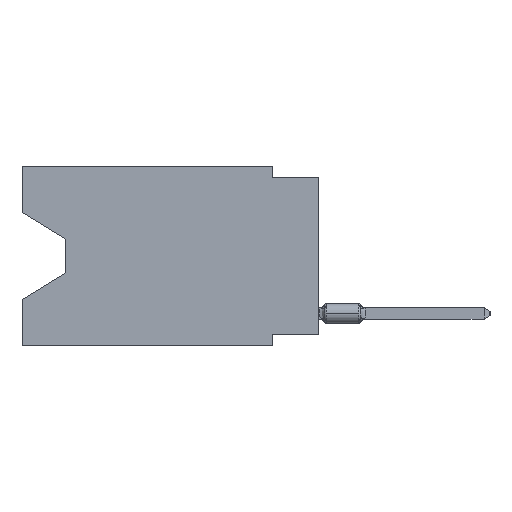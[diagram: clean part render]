
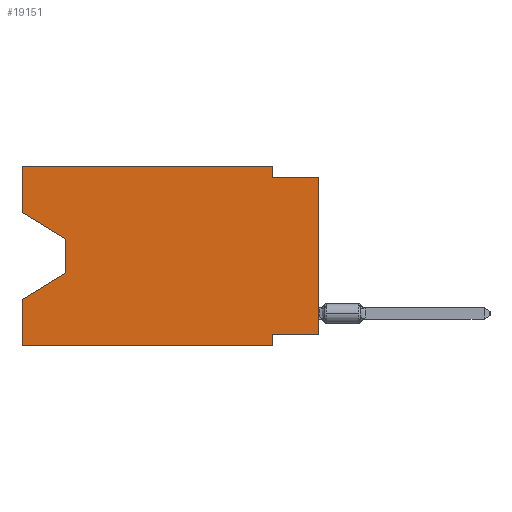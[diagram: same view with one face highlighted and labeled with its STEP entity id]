
A CAD part, left-side view. The second image highlights one B-rep face of the part: STEP entity #19151.
In plain terms, the highlighted planar face has unit normal (-1, 0, 0).
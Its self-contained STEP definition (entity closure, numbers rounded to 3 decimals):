
#124 = CARTESIAN_POINT ( 'NONE',  ( 0., 2.54, -0.635 ) ) ;
#168 = VECTOR ( 'NONE', #8732, 1000. ) ;
#340 = CARTESIAN_POINT ( 'NONE',  ( 0., 2.54, 0. ) ) ;
#761 = CARTESIAN_POINT ( 'NONE',  ( 0., 2.54, -9.271 ) ) ;
#999 = EDGE_CURVE ( 'NONE', #3724, #24567, #1576, .T. ) ;
#1159 = LINE ( 'NONE', #17522, #9940 ) ;
#1576 = LINE ( 'NONE', #15532, #2021 ) ;
#2021 = VECTOR ( 'NONE', #21964, 1000. ) ;
#2259 = VECTOR ( 'NONE', #9205, 1000. ) ;
#2553 = CARTESIAN_POINT ( 'NONE',  ( 0., 16.383, 0. ) ) ;
#3724 = VERTEX_POINT ( 'NONE', #340 ) ;
#3822 = VERTEX_POINT ( 'NONE', #23517 ) ;
#3985 = CARTESIAN_POINT ( 'NONE',  ( 0., 13.97, -4.013 ) ) ;
#4241 = EDGE_CURVE ( 'NONE', #12847, #3724, #4592, .T. ) ;
#4518 = CARTESIAN_POINT ( 'NONE',  ( 0., 16.383, 0. ) ) ;
#4592 = LINE ( 'NONE', #2553, #168 ) ;
#4938 = AXIS2_PLACEMENT_3D ( 'NONE', #4518, #24646, #8543 ) ;
#5073 = VERTEX_POINT ( 'NONE', #761 ) ;
#5089 = EDGE_CURVE ( 'NONE', #18502, #16175, #13225, .T. ) ;
#5400 = EDGE_CURVE ( 'NONE', #19170, #5073, #24892, .T. ) ;
#6096 = DIRECTION ( 'NONE',  ( 0., -0.855, -0.519 ) ) ;
#6120 = DIRECTION ( 'NONE',  ( 0., 0., -1. ) ) ;
#6933 = VECTOR ( 'NONE', #7086, 1000. ) ;
#7086 = DIRECTION ( 'NONE',  ( 0., -1., 0. ) ) ;
#7178 = EDGE_LOOP ( 'NONE', ( #16000, #24976, #16174, #12053, #7689, #14075, #20130, #25928, #21054, #15709, #17109, #22818 ) ) ;
#7386 = CARTESIAN_POINT ( 'NONE',  ( 0., 16.383, 0. ) ) ;
#7527 = VECTOR ( 'NONE', #6096, 1000. ) ;
#7684 = DIRECTION ( 'NONE',  ( 0., -1., 0. ) ) ;
#7689 = ORIENTED_EDGE ( 'NONE', *, *, #8648, .T. ) ;
#8277 = PLANE ( 'NONE',  #4938 ) ;
#8543 = DIRECTION ( 'NONE',  ( 0., 0., -1. ) ) ;
#8648 = EDGE_CURVE ( 'NONE', #18502, #16635, #19505, .T. ) ;
#8732 = DIRECTION ( 'NONE',  ( 0., -1., 0. ) ) ;
#9083 = LINE ( 'NONE', #25455, #6933 ) ;
#9205 = DIRECTION ( 'NONE',  ( 0., 0., 1. ) ) ;
#9466 = CARTESIAN_POINT ( 'NONE',  ( 0., 16.383, 0. ) ) ;
#9786 = CARTESIAN_POINT ( 'NONE',  ( 0., 0., 0. ) ) ;
#9940 = VECTOR ( 'NONE', #11191, 1000. ) ;
#9993 = LINE ( 'NONE', #14555, #7527 ) ;
#11191 = DIRECTION ( 'NONE',  ( 0., 0., 1. ) ) ;
#11523 = DIRECTION ( 'NONE',  ( 0., 0., 1. ) ) ;
#11821 = CARTESIAN_POINT ( 'NONE',  ( 0., 16.383, -9.906 ) ) ;
#12053 = ORIENTED_EDGE ( 'NONE', *, *, #5089, .F. ) ;
#12278 = EDGE_CURVE ( 'NONE', #24567, #22114, #9083, .T. ) ;
#12280 = EDGE_CURVE ( 'NONE', #24946, #16175, #23456, .T. ) ;
#12535 = EDGE_CURVE ( 'NONE', #22841, #12847, #1159, .T. ) ;
#12847 = VERTEX_POINT ( 'NONE', #7386 ) ;
#13225 = LINE ( 'NONE', #9466, #2259 ) ;
#13651 = DIRECTION ( 'NONE',  ( 0., 0.855, -0.519 ) ) ;
#13771 = CARTESIAN_POINT ( 'NONE',  ( 0., 13.97, -5.893 ) ) ;
#14075 = ORIENTED_EDGE ( 'NONE', *, *, #21015, .F. ) ;
#14244 = VECTOR ( 'NONE', #13651, 1000. ) ;
#14555 = CARTESIAN_POINT ( 'NONE',  ( 0., 16.383, -2.546 ) ) ;
#15532 = CARTESIAN_POINT ( 'NONE',  ( 0., 2.54, 0. ) ) ;
#15672 = CARTESIAN_POINT ( 'NONE',  ( 0., 0., -0.635 ) ) ;
#15709 = ORIENTED_EDGE ( 'NONE', *, *, #999, .F. ) ;
#16000 = ORIENTED_EDGE ( 'NONE', *, *, #19570, .T. ) ;
#16169 = CARTESIAN_POINT ( 'NONE',  ( 0., 2.54, -9.906 ) ) ;
#16174 = ORIENTED_EDGE ( 'NONE', *, *, #12280, .T. ) ;
#16175 = VERTEX_POINT ( 'NONE', #18248 ) ;
#16287 = LINE ( 'NONE', #16169, #22493 ) ;
#16613 = FACE_OUTER_BOUND ( 'NONE', #7178, .T. ) ;
#16635 = VERTEX_POINT ( 'NONE', #26372 ) ;
#17109 = ORIENTED_EDGE ( 'NONE', *, *, #4241, .F. ) ;
#17522 = CARTESIAN_POINT ( 'NONE',  ( 0., 16.383, 0. ) ) ;
#17705 = LINE ( 'NONE', #9786, #21175 ) ;
#18248 = CARTESIAN_POINT ( 'NONE',  ( 0., 16.383, -7.36 ) ) ;
#18502 = VERTEX_POINT ( 'NONE', #11821 ) ;
#18803 = CARTESIAN_POINT ( 'NONE',  ( 0., 16.383, -2.546 ) ) ;
#19151 = ADVANCED_FACE ( 'NONE', ( #16613 ), #8277, .F. ) ;
#19170 = VERTEX_POINT ( 'NONE', #22644 ) ;
#19505 = LINE ( 'NONE', #21508, #19817 ) ;
#19570 = EDGE_CURVE ( 'NONE', #22841, #3822, #9993, .T. ) ;
#19817 = VECTOR ( 'NONE', #7684, 1000. ) ;
#20130 = ORIENTED_EDGE ( 'NONE', *, *, #5400, .F. ) ;
#21015 = EDGE_CURVE ( 'NONE', #5073, #16635, #16287, .T. ) ;
#21054 = ORIENTED_EDGE ( 'NONE', *, *, #12278, .F. ) ;
#21175 = VECTOR ( 'NONE', #11523, 1000. ) ;
#21265 = VECTOR ( 'NONE', #6120, 1000. ) ;
#21508 = CARTESIAN_POINT ( 'NONE',  ( 0., 16.383, -9.906 ) ) ;
#21964 = DIRECTION ( 'NONE',  ( 0., 0., -1. ) ) ;
#22114 = VERTEX_POINT ( 'NONE', #15672 ) ;
#22451 = DIRECTION ( 'NONE',  ( 0., 0., -1. ) ) ;
#22493 = VECTOR ( 'NONE', #22451, 1000. ) ;
#22644 = CARTESIAN_POINT ( 'NONE',  ( 0., 0., -9.271 ) ) ;
#22760 = CARTESIAN_POINT ( 'NONE',  ( 0., 0., -9.271 ) ) ;
#22818 = ORIENTED_EDGE ( 'NONE', *, *, #12535, .F. ) ;
#22841 = VERTEX_POINT ( 'NONE', #18803 ) ;
#23109 = EDGE_CURVE ( 'NONE', #19170, #22114, #17705, .T. ) ;
#23263 = VECTOR ( 'NONE', #24643, 1000. ) ;
#23456 = LINE ( 'NONE', #13771, #14244 ) ;
#23517 = CARTESIAN_POINT ( 'NONE',  ( 0., 13.97, -4.013 ) ) ;
#24490 = LINE ( 'NONE', #3985, #21265 ) ;
#24567 = VERTEX_POINT ( 'NONE', #124 ) ;
#24643 = DIRECTION ( 'NONE',  ( 0., 1., 0. ) ) ;
#24646 = DIRECTION ( 'NONE',  ( 1., 0., 0. ) ) ;
#24865 = EDGE_CURVE ( 'NONE', #3822, #24946, #24490, .T. ) ;
#24884 = CARTESIAN_POINT ( 'NONE',  ( 0., 13.97, -5.893 ) ) ;
#24892 = LINE ( 'NONE', #22760, #23263 ) ;
#24946 = VERTEX_POINT ( 'NONE', #24884 ) ;
#24976 = ORIENTED_EDGE ( 'NONE', *, *, #24865, .T. ) ;
#25455 = CARTESIAN_POINT ( 'NONE',  ( 0., 0., -0.635 ) ) ;
#25928 = ORIENTED_EDGE ( 'NONE', *, *, #23109, .T. ) ;
#26372 = CARTESIAN_POINT ( 'NONE',  ( 0., 2.54, -9.906 ) ) ;
